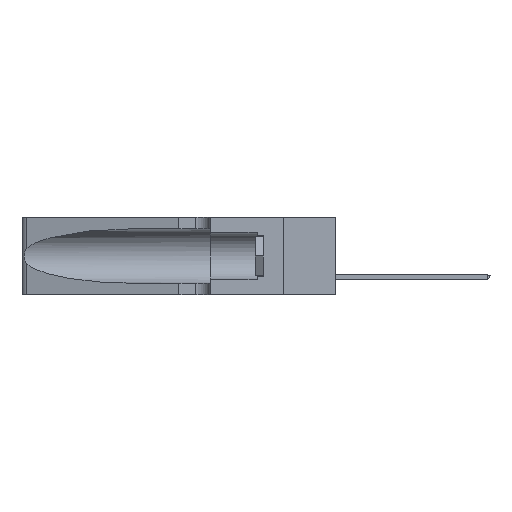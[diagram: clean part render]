
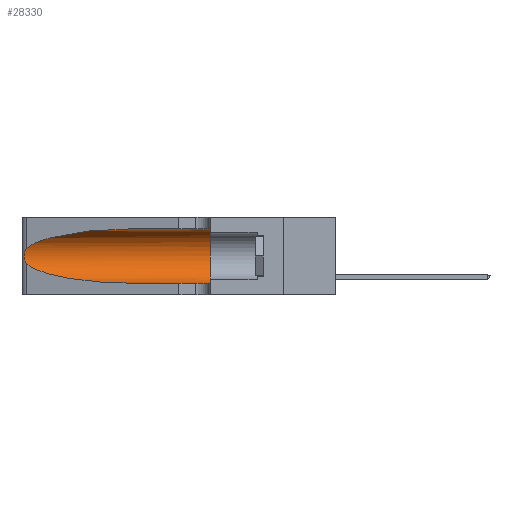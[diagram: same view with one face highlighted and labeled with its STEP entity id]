
A CAD part, left-side view. The second image highlights one B-rep face of the part: STEP entity #28330.
In plain terms, the highlighted cylindrical face has radius 3.308 mm (diameter 6.617 mm), a partial arc.
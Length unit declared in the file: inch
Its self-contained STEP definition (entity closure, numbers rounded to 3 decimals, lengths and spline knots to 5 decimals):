
#1101 = CARTESIAN_POINT ( 'NONE',  ( 0.25787, 1.23484, 0.2124 ) ) ;
#1511 = DIRECTION ( 'NONE',  ( 0., -1., 0. ) ) ;
#1614 = EDGE_CURVE ( 'NONE', #2975, #20411, #26048, .T. ) ;
#1876 = CARTESIAN_POINT ( 'NONE',  ( 0.1305, 0.72297, 0.31525 ) ) ;
#2680 = ORIENTED_EDGE ( 'NONE', *, *, #32337, .T. ) ;
#2975 = VERTEX_POINT ( 'NONE', #24696 ) ;
#3816 = CARTESIAN_POINT ( 'NONE',  ( 0.26018, 1.23835, 0.19895 ) ) ;
#4179 = CARTESIAN_POINT ( 'NONE',  ( 0.18966, 0.96281, 0.31525 ) ) ;
#4200 = ORIENTED_EDGE ( 'NONE', *, *, #1614, .T. ) ;
#4357 = CARTESIAN_POINT ( 'NONE',  ( 0.1305, 1.61858, 0.185 ) ) ;
#4683 = CARTESIAN_POINT ( 'NONE',  ( 0.1305, 0.35, 0.185 ) ) ;
#7643 = CARTESIAN_POINT ( 'NONE',  ( 0.25555, 1.22994, 0.2215 ) ) ;
#8033 = VERTEX_POINT ( 'NONE', #20341 ) ;
#8469 = VECTOR ( 'NONE', #1511, 39.37008 ) ;
#10111 = CARTESIAN_POINT ( 'NONE',  ( 0.1305, 1.61858, 0.31525 ) ) ;
#10338 = CARTESIAN_POINT ( 'NONE',  ( 0.25487, 1.22718, 0.14631 ) ) ;
#10383 = DIRECTION ( 'NONE',  ( 0., -1., 0. ) ) ;
#10611 = DIRECTION ( 'NONE',  ( 0., 0., -1. ) ) ;
#10765 = CARTESIAN_POINT ( 'NONE',  ( 0.26017, 1.23833, 0.17102 ) ) ;
#11671 = VERTEX_POINT ( 'NONE', #34674 ) ;
#12145 = AXIS2_PLACEMENT_3D ( 'NONE', #4357, #30387, #10611 ) ;
#14258 = CARTESIAN_POINT ( 'NONE',  ( 0.1305, 0.72297, 0.31525 ) ) ;
#14401 = CARTESIAN_POINT ( 'NONE',  ( 0.2373, 1.15595, 0.28018 ) ) ;
#15001 = ORIENTED_EDGE ( 'NONE', *, *, #18354, .T. ) ;
#15048 = DIRECTION ( 'NONE',  ( 0., 0., 1. ) ) ;
#15476 = EDGE_LOOP ( 'NONE', ( #2680, #25047, #4200, #15001, #20306, #22161 ) ) ;
#15743 = AXIS2_PLACEMENT_3D ( 'NONE', #4683, #34571, #15048 ) ;
#16721 = CARTESIAN_POINT ( 'NONE',  ( 0.25854, 1.2359, 0.20912 ) ) ;
#17152 = CARTESIAN_POINT ( 'NONE',  ( 0.25639, 1.23184, 0.21858 ) ) ;
#17280 = CARTESIAN_POINT ( 'NONE',  ( 0.25789, 1.23486, 0.15765 ) ) ;
#17830 = CARTESIAN_POINT ( 'NONE',  ( 0.1305, 1.61858, 0.05475 ) ) ;
#18354 = EDGE_CURVE ( 'NONE', #20411, #11671, #21197, .T. ) ;
#18993 = FACE_OUTER_BOUND ( 'NONE', #15476, .T. ) ;
#20143 = EDGE_CURVE ( 'NONE', #23850, #11671, #30257, .T. ) ;
#20291 = CARTESIAN_POINT ( 'NONE',  ( 0.25487, 1.22718, 0.22369 ) ) ;
#20306 = ORIENTED_EDGE ( 'NONE', *, *, #20143, .F. ) ;
#20341 = CARTESIAN_POINT ( 'NONE',  ( 0.25487, 1.22718, 0.22369 ) ) ;
#20411 = VERTEX_POINT ( 'NONE', #41867 ) ;
#20514 = CARTESIAN_POINT ( 'NONE',  ( 0.25487, 1.22718, 0.22369 ) ) ;
#21074 = EDGE_CURVE ( 'NONE', #22236, #23850, #28179, .T. ) ;
#21197 = LINE ( 'NONE', #17830, #8469 ) ;
#22161 = ORIENTED_EDGE ( 'NONE', *, *, #21074, .F. ) ;
#22236 = VERTEX_POINT ( 'NONE', #1876 ) ;
#22714 = CARTESIAN_POINT ( 'NONE',  ( 0.1305, 0.72297, 0.05475 ) ) ;
#23836 = CARTESIAN_POINT ( 'NONE',  ( 0.25555, 1.22993, 0.14849 ) ) ;
#23850 = VERTEX_POINT ( 'NONE', #28997 ) ;
#24696 = CARTESIAN_POINT ( 'NONE',  ( 0.25487, 1.22718, 0.14631 ) ) ;
#25047 = ORIENTED_EDGE ( 'NONE', *, *, #39480, .T. ) ;
#26048 =( BOUNDED_CURVE ( )  B_SPLINE_CURVE ( 3, ( #36138, #29695, #26546, #22714 ),
 .UNSPECIFIED., .F., .T. ) 
 B_SPLINE_CURVE_WITH_KNOTS ( ( 4, 4 ),
 ( 3.44316, 4.71239 ),
 .UNSPECIFIED. ) 
 CURVE ( )  GEOMETRIC_REPRESENTATION_ITEM ( )  RATIONAL_B_SPLINE_CURVE ( ( 1., 0.87, 0.87, 1. ) ) 
 REPRESENTATION_ITEM ( '' )  );
#26546 = CARTESIAN_POINT ( 'NONE',  ( 0.18966, 0.96281, 0.05475 ) ) ;
#26570 = CARTESIAN_POINT ( 'NONE',  ( 0.26075, 1.23896, 0.178 ) ) ;
#26841 =( BOUNDED_CURVE ( )  B_SPLINE_CURVE ( 3, ( #14258, #4179, #14401, #20514 ),
 .UNSPECIFIED., .F., .F. ) 
 B_SPLINE_CURVE_WITH_KNOTS ( ( 4, 4 ),
 ( 1.5708, 2.84003 ),
 .UNSPECIFIED. ) 
 CURVE ( )  GEOMETRIC_REPRESENTATION_ITEM ( )  RATIONAL_B_SPLINE_CURVE ( ( 1., 0.87, 0.87, 1. ) ) 
 REPRESENTATION_ITEM ( '' )  );
#28179 = LINE ( 'NONE', #10111, #41458 ) ;
#28330 = ADVANCED_FACE ( 'NONE', ( #18993 ), #36366, .F. ) ;
#28997 = CARTESIAN_POINT ( 'NONE',  ( 0.1305, 0.35, 0.31525 ) ) ;
#29695 = CARTESIAN_POINT ( 'NONE',  ( 0.2373, 1.15595, 0.08982 ) ) ;
#30257 = CIRCLE ( 'NONE', #15743, 0.13025 ) ;
#30387 = DIRECTION ( 'NONE',  ( 0., -1., 0. ) ) ;
#32337 = EDGE_CURVE ( 'NONE', #22236, #8033, #26841, .T. ) ;
#33540 = CARTESIAN_POINT ( 'NONE',  ( 0.25856, 1.23593, 0.16098 ) ) ;
#33864 = B_SPLINE_CURVE_WITH_KNOTS ( 'NONE', 3,
 ( #20291, #7643, #17152, #1101, #16721, #3816, #39995, #26570, #10765, #33540, #17280, #40128, #23836, #10338 ),
 .UNSPECIFIED., .F., .F.,
 ( 4, 2, 2, 2, 2, 2, 4 ),
 ( 0., 0.00027, 0.00053, 0.00107, 0.0016, 0.00187, 0.00214 ),
 .UNSPECIFIED. ) ;
#34571 = DIRECTION ( 'NONE',  ( 0., 1., 0. ) ) ;
#34674 = CARTESIAN_POINT ( 'NONE',  ( 0.1305, 0.35, 0.05475 ) ) ;
#36138 = CARTESIAN_POINT ( 'NONE',  ( 0.25487, 1.22718, 0.14631 ) ) ;
#36366 = CYLINDRICAL_SURFACE ( 'NONE', #12145, 0.13025 ) ;
#39480 = EDGE_CURVE ( 'NONE', #8033, #2975, #33864, .T. ) ;
#39995 = CARTESIAN_POINT ( 'NONE',  ( 0.26075, 1.23896, 0.19203 ) ) ;
#40128 = CARTESIAN_POINT ( 'NONE',  ( 0.25639, 1.23186, 0.15144 ) ) ;
#41458 = VECTOR ( 'NONE', #10383, 39.37008 ) ;
#41867 = CARTESIAN_POINT ( 'NONE',  ( 0.1305, 0.72297, 0.05475 ) ) ;
